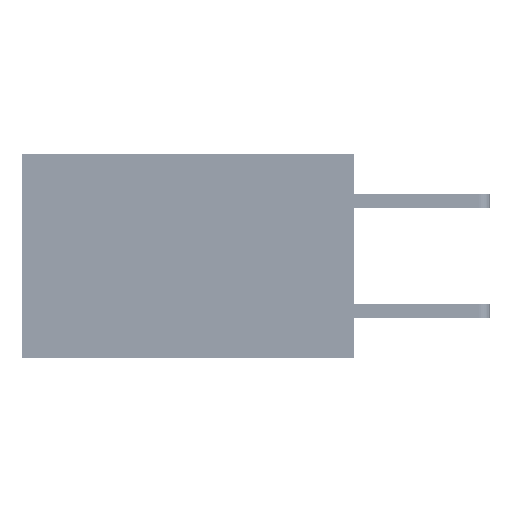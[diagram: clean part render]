
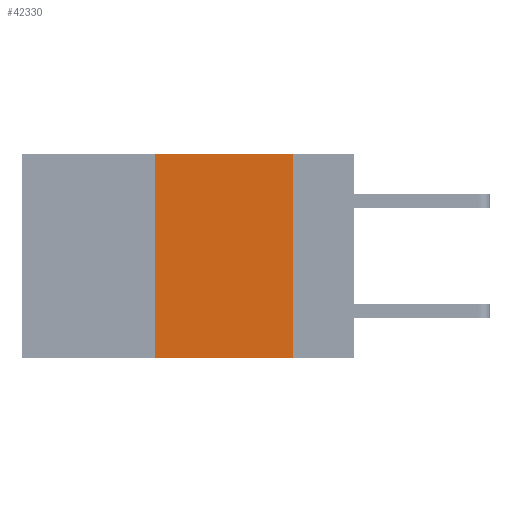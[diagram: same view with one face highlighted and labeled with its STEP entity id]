
A CAD part, left-side view. The second image highlights one B-rep face of the part: STEP entity #42330.
In plain terms, the highlighted planar face has unit normal (-1, 0, 0).
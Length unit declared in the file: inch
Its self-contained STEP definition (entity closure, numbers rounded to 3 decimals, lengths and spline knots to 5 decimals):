
#191 = ORIENTED_EDGE ( 'NONE', *, *, #25488, .F. ) ;
#795 = VECTOR ( 'NONE', #6004, 39.37008 ) ;
#832 = CARTESIAN_POINT ( 'NONE',  ( 0., 0.36, 0. ) ) ;
#1211 = LINE ( 'NONE', #38192, #45485 ) ;
#1978 = DIRECTION ( 'NONE',  ( 0., 0., -1. ) ) ;
#5414 = CARTESIAN_POINT ( 'NONE',  ( 0., 0.11, -0.37 ) ) ;
#5741 = PLANE ( 'NONE',  #44601 ) ;
#5840 = CARTESIAN_POINT ( 'NONE',  ( 0., 0.11, 0. ) ) ;
#6004 = DIRECTION ( 'NONE',  ( 0., 0., 1. ) ) ;
#6012 = CARTESIAN_POINT ( 'NONE',  ( 0., 0.6, 0. ) ) ;
#10349 = VERTEX_POINT ( 'NONE', #832 ) ;
#11540 = LINE ( 'NONE', #43442, #15965 ) ;
#13927 = LINE ( 'NONE', #5840, #38977 ) ;
#15202 = ORIENTED_EDGE ( 'NONE', *, *, #34169, .F. ) ;
#15965 = VECTOR ( 'NONE', #31368, 39.37008 ) ;
#18240 = ORIENTED_EDGE ( 'NONE', *, *, #21812, .F. ) ;
#21234 = EDGE_LOOP ( 'NONE', ( #15202, #18240, #191, #49537 ) ) ;
#21812 = EDGE_CURVE ( 'NONE', #10349, #31337, #11540, .T. ) ;
#22401 = DIRECTION ( 'NONE',  ( 1., 0., 0. ) ) ;
#25488 = EDGE_CURVE ( 'NONE', #35031, #10349, #41950, .T. ) ;
#26233 = DIRECTION ( 'NONE',  ( 0., 0., -1. ) ) ;
#27046 = CARTESIAN_POINT ( 'NONE',  ( 0., 0.36, -0.37 ) ) ;
#27712 = EDGE_CURVE ( 'NONE', #35031, #50611, #1211, .T. ) ;
#30422 = DIRECTION ( 'NONE',  ( 0., -1., 0. ) ) ;
#31337 = VERTEX_POINT ( 'NONE', #33681 ) ;
#31368 = DIRECTION ( 'NONE',  ( 0., -1., 0. ) ) ;
#33681 = CARTESIAN_POINT ( 'NONE',  ( 0., 0.11, 0. ) ) ;
#33899 = CARTESIAN_POINT ( 'NONE',  ( 0., 0.36, 0. ) ) ;
#34169 = EDGE_CURVE ( 'NONE', #31337, #50611, #13927, .T. ) ;
#35031 = VERTEX_POINT ( 'NONE', #27046 ) ;
#38192 = CARTESIAN_POINT ( 'NONE',  ( 0., 0.6, -0.37 ) ) ;
#38977 = VECTOR ( 'NONE', #26233, 39.37008 ) ;
#41950 = LINE ( 'NONE', #33899, #795 ) ;
#42330 = ADVANCED_FACE ( 'NONE', ( #42473 ), #5741, .F. ) ;
#42473 = FACE_OUTER_BOUND ( 'NONE', #21234, .T. ) ;
#43442 = CARTESIAN_POINT ( 'NONE',  ( 0., 0.6, 0. ) ) ;
#44601 = AXIS2_PLACEMENT_3D ( 'NONE', #6012, #22401, #1978 ) ;
#45485 = VECTOR ( 'NONE', #30422, 39.37008 ) ;
#49537 = ORIENTED_EDGE ( 'NONE', *, *, #27712, .T. ) ;
#50611 = VERTEX_POINT ( 'NONE', #5414 ) ;
